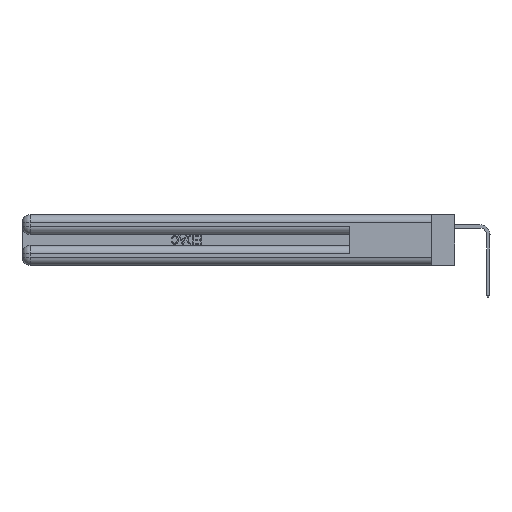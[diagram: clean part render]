
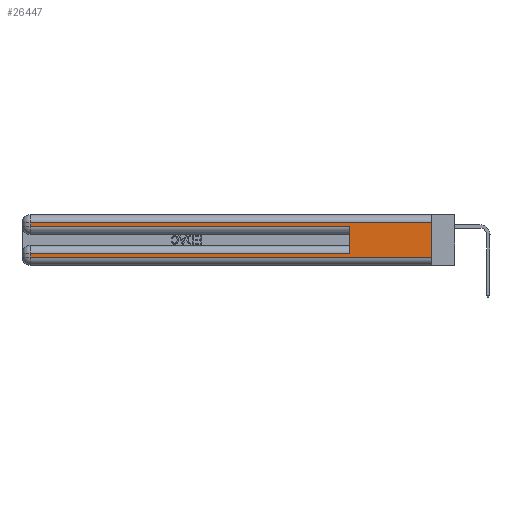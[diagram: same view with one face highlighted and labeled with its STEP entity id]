
A CAD part, left-side view. The second image highlights one B-rep face of the part: STEP entity #26447.
In plain terms, the highlighted planar face has unit normal (-1, 0, 0).
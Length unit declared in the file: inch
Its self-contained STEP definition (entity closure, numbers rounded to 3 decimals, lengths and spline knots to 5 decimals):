
#789 = LINE ( 'NONE', #13044, #13387 ) ;
#908 = VERTEX_POINT ( 'NONE', #53550 ) ;
#4566 = VECTOR ( 'NONE', #39624, 39.37008 ) ;
#5342 = ORIENTED_EDGE ( 'NONE', *, *, #33286, .F. ) ;
#5873 = LINE ( 'NONE', #17456, #36678 ) ;
#6126 = CARTESIAN_POINT ( 'NONE',  ( 0., 0.6, 0.145 ) ) ;
#7255 = CARTESIAN_POINT ( 'NONE',  ( 0., 0.6, 0.285 ) ) ;
#7475 = AXIS2_PLACEMENT_3D ( 'NONE', #46665, #21624, #50845 ) ;
#8421 = DIRECTION ( 'NONE',  ( 0., 0., -1. ) ) ;
#10872 = EDGE_CURVE ( 'NONE', #46534, #20989, #789, .T. ) ;
#10897 = ORIENTED_EDGE ( 'NONE', *, *, #22428, .T. ) ;
#11576 = FACE_OUTER_BOUND ( 'NONE', #17801, .T. ) ;
#12318 = LINE ( 'NONE', #27733, #44322 ) ;
#13044 = CARTESIAN_POINT ( 'NONE',  ( 0., 0., 0.285 ) ) ;
#13229 = PLANE ( 'NONE',  #7475 ) ;
#13387 = VECTOR ( 'NONE', #42260, 39.37008 ) ;
#13664 = EDGE_CURVE ( 'NONE', #22049, #40523, #12318, .T. ) ;
#14898 = VERTEX_POINT ( 'NONE', #33115 ) ;
#14982 = CARTESIAN_POINT ( 'NONE',  ( 0., 2.94, 0.37 ) ) ;
#16635 = ORIENTED_EDGE ( 'NONE', *, *, #48324, .T. ) ;
#17090 = LINE ( 'NONE', #6126, #4566 ) ;
#17456 = CARTESIAN_POINT ( 'NONE',  ( 0., 0., 0.085 ) ) ;
#17499 = EDGE_CURVE ( 'NONE', #46931, #41164, #5873, .T. ) ;
#17801 = EDGE_LOOP ( 'NONE', ( #5342, #42717, #16635, #42771, #52603, #48119, #10897, #33191 ) ) ;
#19344 = DIRECTION ( 'NONE',  ( 0., 1., 0. ) ) ;
#20931 = CARTESIAN_POINT ( 'NONE',  ( 0., 0., 0.37 ) ) ;
#20989 = VERTEX_POINT ( 'NONE', #7255 ) ;
#21624 = DIRECTION ( 'NONE',  ( 1., 0., 0. ) ) ;
#22049 = VERTEX_POINT ( 'NONE', #46900 ) ;
#22428 = EDGE_CURVE ( 'NONE', #41164, #14898, #26986, .T. ) ;
#26447 = ADVANCED_FACE ( 'NONE', ( #11576 ), #13229, .F. ) ;
#26986 = LINE ( 'NONE', #30861, #28317 ) ;
#27258 = CARTESIAN_POINT ( 'NONE',  ( 0., 2.94, 0.31 ) ) ;
#27324 = DIRECTION ( 'NONE',  ( 0., -1., 0. ) ) ;
#27733 = CARTESIAN_POINT ( 'NONE',  ( 0., 0., 0.31 ) ) ;
#28317 = VECTOR ( 'NONE', #47511, 39.37008 ) ;
#29030 = CARTESIAN_POINT ( 'NONE',  ( 0., 0.6, 0.085 ) ) ;
#29755 = EDGE_CURVE ( 'NONE', #14898, #908, #47239, .T. ) ;
#29961 = VECTOR ( 'NONE', #44227, 39.37008 ) ;
#30066 = DIRECTION ( 'NONE',  ( 0., 1., 0. ) ) ;
#30861 = CARTESIAN_POINT ( 'NONE',  ( 0., 2.94, 0.37 ) ) ;
#30887 = CARTESIAN_POINT ( 'NONE',  ( 0., 2.94, 0.285 ) ) ;
#33115 = CARTESIAN_POINT ( 'NONE',  ( 0., 2.94, 0.06 ) ) ;
#33191 = ORIENTED_EDGE ( 'NONE', *, *, #29755, .T. ) ;
#33286 = EDGE_CURVE ( 'NONE', #22049, #908, #46265, .T. ) ;
#35109 = VECTOR ( 'NONE', #8421, 39.37008 ) ;
#36678 = VECTOR ( 'NONE', #30066, 39.37008 ) ;
#39624 = DIRECTION ( 'NONE',  ( 0., 0., 1. ) ) ;
#39744 = LINE ( 'NONE', #14982, #29961 ) ;
#40523 = VERTEX_POINT ( 'NONE', #27258 ) ;
#41164 = VERTEX_POINT ( 'NONE', #44796 ) ;
#42260 = DIRECTION ( 'NONE',  ( 0., -1., 0. ) ) ;
#42717 = ORIENTED_EDGE ( 'NONE', *, *, #13664, .T. ) ;
#42771 = ORIENTED_EDGE ( 'NONE', *, *, #10872, .T. ) ;
#44227 = DIRECTION ( 'NONE',  ( 0., 0., -1. ) ) ;
#44322 = VECTOR ( 'NONE', #19344, 39.37008 ) ;
#44796 = CARTESIAN_POINT ( 'NONE',  ( 0., 2.94, 0.085 ) ) ;
#45929 = VECTOR ( 'NONE', #27324, 39.37008 ) ;
#46265 = LINE ( 'NONE', #20931, #35109 ) ;
#46534 = VERTEX_POINT ( 'NONE', #30887 ) ;
#46585 = EDGE_CURVE ( 'NONE', #46931, #20989, #17090, .T. ) ;
#46665 = CARTESIAN_POINT ( 'NONE',  ( 0., 0., 0.37 ) ) ;
#46900 = CARTESIAN_POINT ( 'NONE',  ( 0., 0., 0.31 ) ) ;
#46931 = VERTEX_POINT ( 'NONE', #29030 ) ;
#47239 = LINE ( 'NONE', #48186, #45929 ) ;
#47511 = DIRECTION ( 'NONE',  ( 0., 0., -1. ) ) ;
#48119 = ORIENTED_EDGE ( 'NONE', *, *, #17499, .T. ) ;
#48186 = CARTESIAN_POINT ( 'NONE',  ( 0., 0., 0.06 ) ) ;
#48324 = EDGE_CURVE ( 'NONE', #40523, #46534, #39744, .T. ) ;
#50845 = DIRECTION ( 'NONE',  ( 0., 0., -1. ) ) ;
#52603 = ORIENTED_EDGE ( 'NONE', *, *, #46585, .F. ) ;
#53550 = CARTESIAN_POINT ( 'NONE',  ( 0., 0., 0.06 ) ) ;
